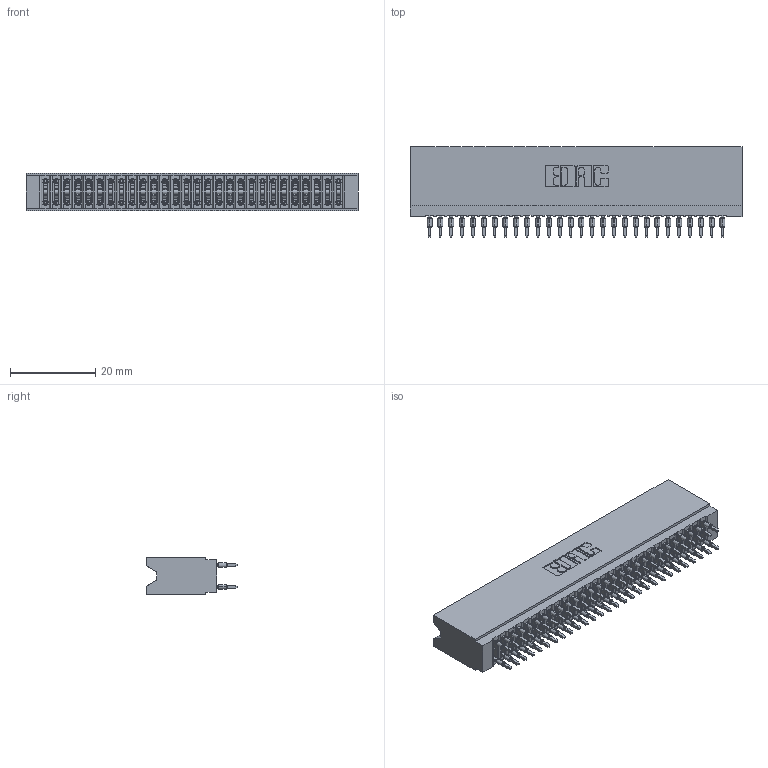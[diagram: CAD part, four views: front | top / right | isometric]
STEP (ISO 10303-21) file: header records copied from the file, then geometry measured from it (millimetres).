
FILE_DESCRIPTION (( 'STEP AP203' ), '1' );
FILE_NAME ('745-056-560-206.STEP', '2026-02-26T18:45:10', ( '' ), ( '' ), 'SwSTEP 2.0', 'SolidWorks 2023', '' );
FILE_SCHEMA (( 'CONFIG_CONTROL_DESIGN' ));
Length unit declared in the file: millimetre
Products named in the file (3): 745-056-560-206; 745-292-001_560; 745 Part_Insulator Option - 06
Assembly tree (57 placements, depth 2):
  745-056-560-206
    745 Part_Insulator Option - 06
    745-292-001_560  x56
Bounding box: 77.72 x 21.22 x 8.89 mm (x, y, z)
Volume: 7268.9 mm3; surface area: 15363.5 mm2
Topology: 57 solids, 57 shells, 5612 faces, 15352 edges, 9748 vertices
Faces by surface type: plane 2912, cylinder 1244, bspline 1120, torus 336
Entity records: 49393 total; most frequent: CARTESIAN_POINT 9076, ORIENTED_EDGE 8484, DIRECTION 7428, EDGE_CURVE 4242, LINE 3884, VECTOR 3884, VERTEX_POINT 2708, AXIS2_PLACEMENT_3D 1772
